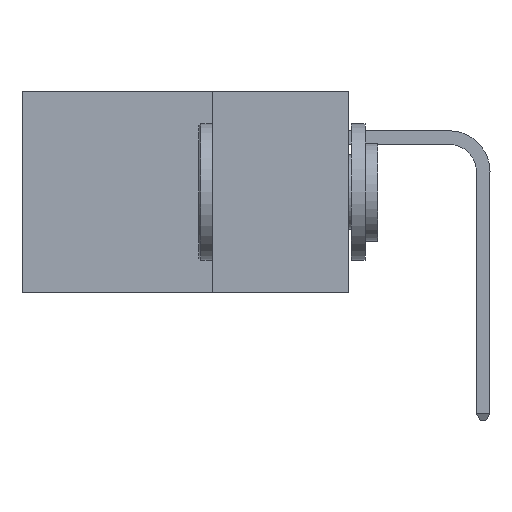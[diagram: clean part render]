
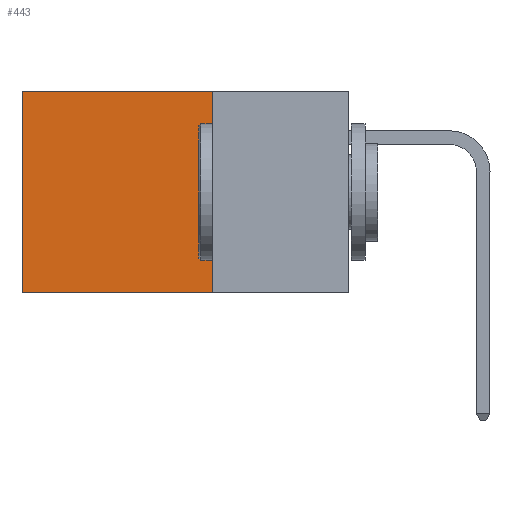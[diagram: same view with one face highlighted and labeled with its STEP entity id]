
A CAD part, left-side view. The second image highlights one B-rep face of the part: STEP entity #443.
In plain terms, the highlighted planar face has unit normal (-1, 0, 0).
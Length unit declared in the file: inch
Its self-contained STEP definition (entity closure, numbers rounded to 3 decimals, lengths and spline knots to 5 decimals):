
#443 = ADVANCED_FACE ( 'NONE', ( #16215 ), #18633, .F. ) ;
#773 = EDGE_LOOP ( 'NONE', ( #4080, #13945, #17075, #9519 ) ) ;
#1788 = VECTOR ( 'NONE', #13934, 39.37008 ) ;
#4080 = ORIENTED_EDGE ( 'NONE', *, *, #10635, .T. ) ;
#4643 = DIRECTION ( 'NONE',  ( 0., 1., 0. ) ) ;
#5600 = EDGE_CURVE ( 'NONE', #12925, #5850, #22250, .T. ) ;
#5850 = VERTEX_POINT ( 'NONE', #21682 ) ;
#6446 = LINE ( 'NONE', #8504, #15121 ) ;
#6991 = CARTESIAN_POINT ( 'NONE',  ( 0.2875, 0.25, 0. ) ) ;
#7276 = AXIS2_PLACEMENT_3D ( 'NONE', #19111, #18590, #18568 ) ;
#8144 = VERTEX_POINT ( 'NONE', #8980 ) ;
#8504 = CARTESIAN_POINT ( 'NONE',  ( 0.2875, 0.6, 0. ) ) ;
#8980 = CARTESIAN_POINT ( 'NONE',  ( 0.2875, 0.6, -0.37 ) ) ;
#9329 = CARTESIAN_POINT ( 'NONE',  ( 0.2875, 0.25, 0. ) ) ;
#9347 = VERTEX_POINT ( 'NONE', #20001 ) ;
#9418 = VECTOR ( 'NONE', #19392, 39.37008 ) ;
#9519 = ORIENTED_EDGE ( 'NONE', *, *, #14567, .T. ) ;
#10635 = EDGE_CURVE ( 'NONE', #9347, #8144, #6446, .T. ) ;
#11350 = LINE ( 'NONE', #22172, #1788 ) ;
#12925 = VERTEX_POINT ( 'NONE', #6991 ) ;
#13934 = DIRECTION ( 'NONE',  ( 0., 1., 0. ) ) ;
#13945 = ORIENTED_EDGE ( 'NONE', *, *, #22459, .F. ) ;
#14567 = EDGE_CURVE ( 'NONE', #12925, #9347, #11350, .T. ) ;
#15092 = CARTESIAN_POINT ( 'NONE',  ( 0.2875, 0.25, -0.37 ) ) ;
#15121 = VECTOR ( 'NONE', #21964, 39.37008 ) ;
#15844 = LINE ( 'NONE', #15092, #20237 ) ;
#16215 = FACE_OUTER_BOUND ( 'NONE', #773, .T. ) ;
#17075 = ORIENTED_EDGE ( 'NONE', *, *, #5600, .F. ) ;
#18568 = DIRECTION ( 'NONE',  ( 0., 0., -1. ) ) ;
#18590 = DIRECTION ( 'NONE',  ( 1., 0., 0. ) ) ;
#18633 = PLANE ( 'NONE',  #7276 ) ;
#19111 = CARTESIAN_POINT ( 'NONE',  ( 0.2875, 0.25, 0. ) ) ;
#19392 = DIRECTION ( 'NONE',  ( 0., 0., -1. ) ) ;
#20001 = CARTESIAN_POINT ( 'NONE',  ( 0.2875, 0.6, 0. ) ) ;
#20237 = VECTOR ( 'NONE', #4643, 39.37008 ) ;
#21682 = CARTESIAN_POINT ( 'NONE',  ( 0.2875, 0.25, -0.37 ) ) ;
#21964 = DIRECTION ( 'NONE',  ( 0., 0., -1. ) ) ;
#22172 = CARTESIAN_POINT ( 'NONE',  ( 0.2875, 0.25, 0. ) ) ;
#22250 = LINE ( 'NONE', #9329, #9418 ) ;
#22459 = EDGE_CURVE ( 'NONE', #5850, #8144, #15844, .T. ) ;
